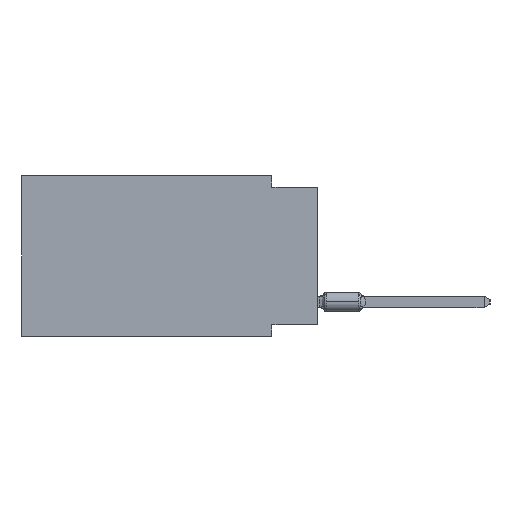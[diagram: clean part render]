
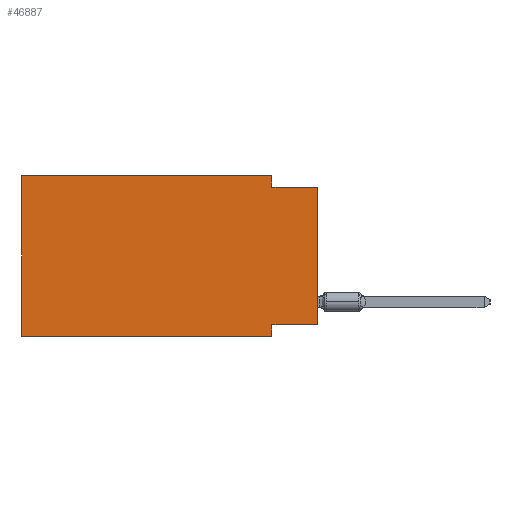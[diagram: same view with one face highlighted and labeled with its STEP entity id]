
A CAD part, left-side view. The second image highlights one B-rep face of the part: STEP entity #46887.
In plain terms, the highlighted planar face has unit normal (-1, 0, 0).
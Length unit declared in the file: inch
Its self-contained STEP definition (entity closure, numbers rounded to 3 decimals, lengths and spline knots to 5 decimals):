
#1086 = DIRECTION ( 'NONE',  ( 0., -1., 0. ) ) ;
#1550 = CARTESIAN_POINT ( 'NONE',  ( 0., 0.1, 0. ) ) ;
#1781 = DIRECTION ( 'NONE',  ( 0., 0., -1. ) ) ;
#3055 = LINE ( 'NONE', #20962, #30102 ) ;
#3689 = EDGE_CURVE ( 'NONE', #7065, #19842, #29770, .T. ) ;
#4048 = CARTESIAN_POINT ( 'NONE',  ( 0., 0.645, 0. ) ) ;
#4791 = VECTOR ( 'NONE', #38164, 39.37008 ) ;
#5101 = AXIS2_PLACEMENT_3D ( 'NONE', #53619, #24642, #1781 ) ;
#5252 = VECTOR ( 'NONE', #1086, 39.37008 ) ;
#6023 = DIRECTION ( 'NONE',  ( 0., 1., 0. ) ) ;
#6801 = LINE ( 'NONE', #53310, #5252 ) ;
#7065 = VERTEX_POINT ( 'NONE', #15029 ) ;
#7114 = FACE_OUTER_BOUND ( 'NONE', #15815, .T. ) ;
#7217 = ORIENTED_EDGE ( 'NONE', *, *, #37150, .F. ) ;
#8620 = LINE ( 'NONE', #4048, #53240 ) ;
#9750 = DIRECTION ( 'NONE',  ( 0., 0., 1. ) ) ;
#9873 = VERTEX_POINT ( 'NONE', #38739 ) ;
#11096 = VERTEX_POINT ( 'NONE', #21222 ) ;
#11341 = CARTESIAN_POINT ( 'NONE',  ( 0., 0., -0.325 ) ) ;
#11718 = VECTOR ( 'NONE', #21647, 39.37008 ) ;
#11824 = DIRECTION ( 'NONE',  ( 0., 0., -1. ) ) ;
#12260 = VECTOR ( 'NONE', #11824, 39.37008 ) ;
#14502 = CARTESIAN_POINT ( 'NONE',  ( 0., 0.1, -0.35 ) ) ;
#15029 = CARTESIAN_POINT ( 'NONE',  ( 0., 0.1, 0. ) ) ;
#15132 = CARTESIAN_POINT ( 'NONE',  ( 0., 0.645, -0.35 ) ) ;
#15815 = EDGE_LOOP ( 'NONE', ( #17765, #7217, #74461, #66075, #30428, #59787, #35740, #60611 ) ) ;
#17765 = ORIENTED_EDGE ( 'NONE', *, *, #59314, .T. ) ;
#19842 = VERTEX_POINT ( 'NONE', #62870 ) ;
#20962 = CARTESIAN_POINT ( 'NONE',  ( 0., 0., 0. ) ) ;
#21222 = CARTESIAN_POINT ( 'NONE',  ( 0., 0.645, 0. ) ) ;
#21467 = VERTEX_POINT ( 'NONE', #49984 ) ;
#21647 = DIRECTION ( 'NONE',  ( 0., -1., 0. ) ) ;
#22394 = CARTESIAN_POINT ( 'NONE',  ( 0., 0., -0.025 ) ) ;
#23495 = EDGE_CURVE ( 'NONE', #9873, #21467, #37635, .T. ) ;
#24642 = DIRECTION ( 'NONE',  ( 1., 0., 0. ) ) ;
#27855 = EDGE_CURVE ( 'NONE', #75201, #21467, #48486, .T. ) ;
#29379 = CARTESIAN_POINT ( 'NONE',  ( 0., 0.1, -0.325 ) ) ;
#29770 = LINE ( 'NONE', #1550, #12260 ) ;
#30102 = VECTOR ( 'NONE', #43835, 39.37008 ) ;
#30359 = PLANE ( 'NONE',  #5101 ) ;
#30428 = ORIENTED_EDGE ( 'NONE', *, *, #59743, .F. ) ;
#34856 = CARTESIAN_POINT ( 'NONE',  ( 0., 0., -0.025 ) ) ;
#35740 = ORIENTED_EDGE ( 'NONE', *, *, #27855, .F. ) ;
#37150 = EDGE_CURVE ( 'NONE', #19842, #70564, #62056, .T. ) ;
#37635 = LINE ( 'NONE', #15132, #61842 ) ;
#38007 = DIRECTION ( 'NONE',  ( 0., -1., 0. ) ) ;
#38164 = DIRECTION ( 'NONE',  ( 0., 0., -1. ) ) ;
#38739 = CARTESIAN_POINT ( 'NONE',  ( 0., 0.645, -0.35 ) ) ;
#40323 = LINE ( 'NONE', #11341, #54155 ) ;
#43835 = DIRECTION ( 'NONE',  ( 0., 0., 1. ) ) ;
#46887 = ADVANCED_FACE ( 'NONE', ( #7114 ), #30359, .F. ) ;
#48486 = LINE ( 'NONE', #14502, #4791 ) ;
#48779 = EDGE_CURVE ( 'NONE', #11096, #7065, #6801, .T. ) ;
#49984 = CARTESIAN_POINT ( 'NONE',  ( 0., 0.1, -0.35 ) ) ;
#53240 = VECTOR ( 'NONE', #9750, 39.37008 ) ;
#53310 = CARTESIAN_POINT ( 'NONE',  ( 0., 0.645, 0. ) ) ;
#53619 = CARTESIAN_POINT ( 'NONE',  ( 0., 0.645, 0. ) ) ;
#54155 = VECTOR ( 'NONE', #6023, 39.37008 ) ;
#55802 = VERTEX_POINT ( 'NONE', #70319 ) ;
#56569 = EDGE_CURVE ( 'NONE', #55802, #75201, #40323, .T. ) ;
#59314 = EDGE_CURVE ( 'NONE', #55802, #70564, #3055, .T. ) ;
#59743 = EDGE_CURVE ( 'NONE', #9873, #11096, #8620, .T. ) ;
#59787 = ORIENTED_EDGE ( 'NONE', *, *, #23495, .T. ) ;
#60611 = ORIENTED_EDGE ( 'NONE', *, *, #56569, .F. ) ;
#61842 = VECTOR ( 'NONE', #38007, 39.37008 ) ;
#62056 = LINE ( 'NONE', #22394, #11718 ) ;
#62870 = CARTESIAN_POINT ( 'NONE',  ( 0., 0.1, -0.025 ) ) ;
#66075 = ORIENTED_EDGE ( 'NONE', *, *, #48779, .F. ) ;
#70319 = CARTESIAN_POINT ( 'NONE',  ( 0., 0., -0.325 ) ) ;
#70564 = VERTEX_POINT ( 'NONE', #34856 ) ;
#74461 = ORIENTED_EDGE ( 'NONE', *, *, #3689, .F. ) ;
#75201 = VERTEX_POINT ( 'NONE', #29379 ) ;
